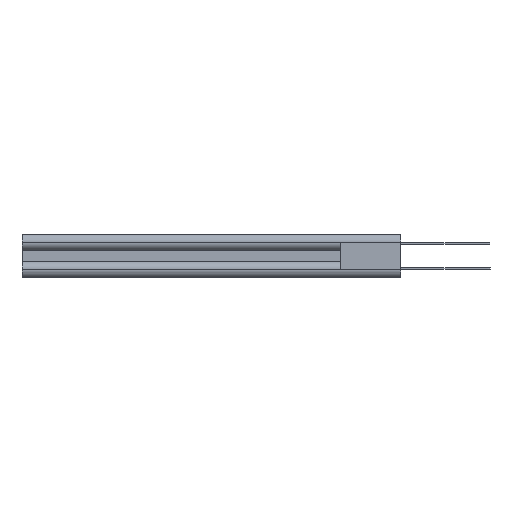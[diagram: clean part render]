
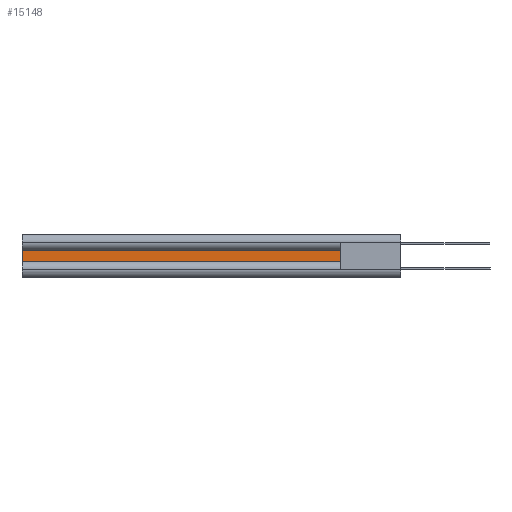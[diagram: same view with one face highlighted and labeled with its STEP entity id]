
A CAD part, left-side view. The second image highlights one B-rep face of the part: STEP entity #15148.
In plain terms, the highlighted planar face has unit normal (-1, 0, 0).
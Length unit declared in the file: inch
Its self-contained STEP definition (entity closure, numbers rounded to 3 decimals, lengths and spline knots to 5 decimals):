
#56 = CARTESIAN_POINT ( 'NONE',  ( 0.044, 0.473, 0.0465 ) ) ;
#587 = VERTEX_POINT ( 'NONE', #56 ) ;
#862 = FACE_OUTER_BOUND ( 'NONE', #15366, .T. ) ;
#884 = EDGE_CURVE ( 'NONE', #587, #9917, #3650, .T. ) ;
#1377 = ORIENTED_EDGE ( 'NONE', *, *, #1392, .T. ) ;
#1392 = EDGE_CURVE ( 'NONE', #587, #19105, #6675, .T. ) ;
#2173 = CARTESIAN_POINT ( 'NONE',  ( 0.044, 0.473, -0.0465 ) ) ;
#3650 = LINE ( 'NONE', #13098, #12364 ) ;
#6675 = LINE ( 'NONE', #19055, #11840 ) ;
#7083 = CARTESIAN_POINT ( 'NONE',  ( 0.044, 3., -0.0465 ) ) ;
#7292 = DIRECTION ( 'NONE',  ( 0., 1., 0. ) ) ;
#7722 = DIRECTION ( 'NONE',  ( 0., 0., -1. ) ) ;
#8329 = CARTESIAN_POINT ( 'NONE',  ( 0.044, 3., -0.0465 ) ) ;
#8360 = ORIENTED_EDGE ( 'NONE', *, *, #9845, .F. ) ;
#8888 = LINE ( 'NONE', #10794, #12915 ) ;
#9845 = EDGE_CURVE ( 'NONE', #9917, #15573, #8888, .T. ) ;
#9917 = VERTEX_POINT ( 'NONE', #2173 ) ;
#10595 = AXIS2_PLACEMENT_3D ( 'NONE', #11066, #17895, #7722 ) ;
#10794 = CARTESIAN_POINT ( 'NONE',  ( 0.044, 0.37012, -0.0465 ) ) ;
#11066 = CARTESIAN_POINT ( 'NONE',  ( 0.044, 0.37012, -0.0465 ) ) ;
#11840 = VECTOR ( 'NONE', #15539, 39.37008 ) ;
#12364 = VECTOR ( 'NONE', #13533, 39.37008 ) ;
#12915 = VECTOR ( 'NONE', #7292, 39.37008 ) ;
#13098 = CARTESIAN_POINT ( 'NONE',  ( 0.044, 0.473, -0.0465 ) ) ;
#13385 = LINE ( 'NONE', #8329, #21183 ) ;
#13533 = DIRECTION ( 'NONE',  ( 0., 0., -1. ) ) ;
#15148 = ADVANCED_FACE ( 'NONE', ( #862 ), #16225, .F. ) ;
#15366 = EDGE_LOOP ( 'NONE', ( #1377, #16826, #8360, #17966 ) ) ;
#15539 = DIRECTION ( 'NONE',  ( 0., 1., 0. ) ) ;
#15573 = VERTEX_POINT ( 'NONE', #7083 ) ;
#15880 = CARTESIAN_POINT ( 'NONE',  ( 0.044, 3., 0.0465 ) ) ;
#16225 = PLANE ( 'NONE',  #10595 ) ;
#16728 = EDGE_CURVE ( 'NONE', #19105, #15573, #13385, .T. ) ;
#16813 = DIRECTION ( 'NONE',  ( 0., 0., -1. ) ) ;
#16826 = ORIENTED_EDGE ( 'NONE', *, *, #16728, .T. ) ;
#17895 = DIRECTION ( 'NONE',  ( 1., 0., 0. ) ) ;
#17966 = ORIENTED_EDGE ( 'NONE', *, *, #884, .F. ) ;
#19055 = CARTESIAN_POINT ( 'NONE',  ( 0.044, 0.37012, 0.0465 ) ) ;
#19105 = VERTEX_POINT ( 'NONE', #15880 ) ;
#21183 = VECTOR ( 'NONE', #16813, 39.37008 ) ;
